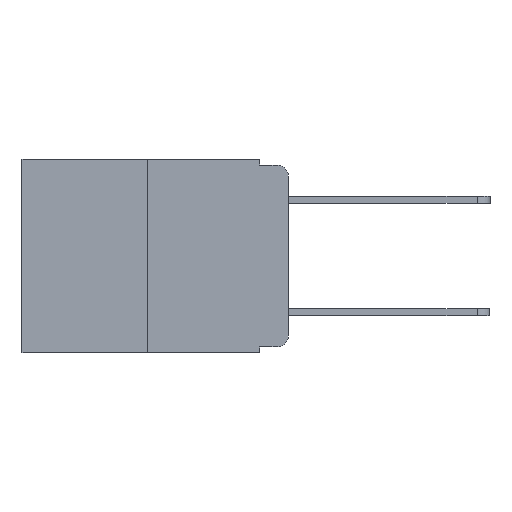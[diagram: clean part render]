
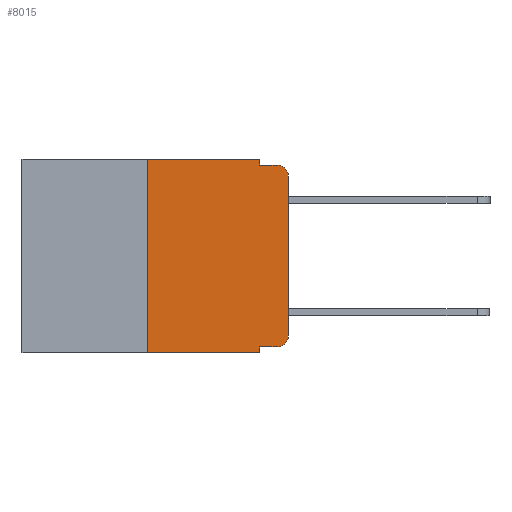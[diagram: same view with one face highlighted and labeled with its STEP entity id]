
A CAD part, left-side view. The second image highlights one B-rep face of the part: STEP entity #8015.
In plain terms, the highlighted planar face has unit normal (-1, 0, 0).
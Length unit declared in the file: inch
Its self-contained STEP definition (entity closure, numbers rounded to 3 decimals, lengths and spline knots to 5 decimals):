
#145 = CARTESIAN_POINT ( 'NONE',  ( 0., 0.02, -0.333 ) ) ;
#206 = DIRECTION ( 'NONE',  ( -1., 0., 0. ) ) ;
#389 = VECTOR ( 'NONE', #14884, 39.37008 ) ;
#493 = EDGE_CURVE ( 'NONE', #17603, #16536, #7752, .T. ) ;
#823 = CARTESIAN_POINT ( 'NONE',  ( 0., 0.051, 0. ) ) ;
#953 = VERTEX_POINT ( 'NONE', #11860 ) ;
#973 = CARTESIAN_POINT ( 'NONE',  ( 0., 0.051, 0. ) ) ;
#1228 = CARTESIAN_POINT ( 'NONE',  ( 0., 0.051, -0.01 ) ) ;
#1438 = LINE ( 'NONE', #3188, #389 ) ;
#1512 = VERTEX_POINT ( 'NONE', #4310 ) ;
#1547 = PLANE ( 'NONE',  #3725 ) ;
#1634 = EDGE_CURVE ( 'NONE', #16536, #2215, #11098, .T. ) ;
#1791 = ORIENTED_EDGE ( 'NONE', *, *, #10806, .T. ) ;
#2012 = VERTEX_POINT ( 'NONE', #9566 ) ;
#2027 = LINE ( 'NONE', #12851, #13285 ) ;
#2215 = VERTEX_POINT ( 'NONE', #7210 ) ;
#2433 = CIRCLE ( 'NONE', #15498, 0.02 ) ;
#2696 = DIRECTION ( 'NONE',  ( 0., 0., -1. ) ) ;
#2817 = LINE ( 'NONE', #3338, #10207 ) ;
#3058 = ORIENTED_EDGE ( 'NONE', *, *, #493, .F. ) ;
#3075 = DIRECTION ( 'NONE',  ( 1., 0., 0. ) ) ;
#3188 = CARTESIAN_POINT ( 'NONE',  ( 0., 0., 0. ) ) ;
#3217 = DIRECTION ( 'NONE',  ( 0., 0., -1. ) ) ;
#3338 = CARTESIAN_POINT ( 'NONE',  ( 0., 0.473, -0.343 ) ) ;
#3560 = EDGE_CURVE ( 'NONE', #15031, #16398, #2027, .T. ) ;
#3725 = AXIS2_PLACEMENT_3D ( 'NONE', #7516, #3075, #13332 ) ;
#3840 = VECTOR ( 'NONE', #14391, 39.37008 ) ;
#4052 = VERTEX_POINT ( 'NONE', #7897 ) ;
#4310 = CARTESIAN_POINT ( 'NONE',  ( 0., 0.02, -0.01 ) ) ;
#4951 = EDGE_CURVE ( 'NONE', #4052, #2012, #2817, .T. ) ;
#5381 = ORIENTED_EDGE ( 'NONE', *, *, #9598, .F. ) ;
#5998 = DIRECTION ( 'NONE',  ( 0., 0., 1. ) ) ;
#7075 = ORIENTED_EDGE ( 'NONE', *, *, #4951, .T. ) ;
#7210 = CARTESIAN_POINT ( 'NONE',  ( 0., 0.051, -0.01 ) ) ;
#7279 = DIRECTION ( 'NONE',  ( -1., 0., 0. ) ) ;
#7516 = CARTESIAN_POINT ( 'NONE',  ( 0., 0.473, 0. ) ) ;
#7700 = VECTOR ( 'NONE', #3217, 39.37008 ) ;
#7752 = LINE ( 'NONE', #12990, #3840 ) ;
#7897 = CARTESIAN_POINT ( 'NONE',  ( 0., 0.25, -0.343 ) ) ;
#8015 = ADVANCED_FACE ( 'NONE', ( #13972 ), #1547, .F. ) ;
#8384 = ORIENTED_EDGE ( 'NONE', *, *, #15509, .T. ) ;
#8617 = ORIENTED_EDGE ( 'NONE', *, *, #1634, .F. ) ;
#8684 = VERTEX_POINT ( 'NONE', #16369 ) ;
#8694 = LINE ( 'NONE', #1228, #12585 ) ;
#8867 = ORIENTED_EDGE ( 'NONE', *, *, #8963, .F. ) ;
#8900 = DIRECTION ( 'NONE',  ( 0., -1., 0. ) ) ;
#8963 = EDGE_CURVE ( 'NONE', #2215, #1512, #8694, .T. ) ;
#9245 = CARTESIAN_POINT ( 'NONE',  ( 0., 0.02, -0.313 ) ) ;
#9375 = LINE ( 'NONE', #10397, #16562 ) ;
#9533 = ORIENTED_EDGE ( 'NONE', *, *, #16787, .T. ) ;
#9566 = CARTESIAN_POINT ( 'NONE',  ( 0., 0.051, -0.343 ) ) ;
#9598 = EDGE_CURVE ( 'NONE', #4052, #17603, #9375, .T. ) ;
#9983 = LINE ( 'NONE', #973, #12927 ) ;
#9994 = DIRECTION ( 'NONE',  ( 0., -1., 0. ) ) ;
#10207 = VECTOR ( 'NONE', #8900, 39.37008 ) ;
#10397 = CARTESIAN_POINT ( 'NONE',  ( 0., 0.25, 0. ) ) ;
#10599 = CARTESIAN_POINT ( 'NONE',  ( 0., 0.051, -0.333 ) ) ;
#10615 = ORIENTED_EDGE ( 'NONE', *, *, #3560, .T. ) ;
#10740 = DIRECTION ( 'NONE',  ( 0., 0., -1. ) ) ;
#10806 = EDGE_CURVE ( 'NONE', #16398, #953, #18041, .T. ) ;
#11098 = LINE ( 'NONE', #823, #7700 ) ;
#11575 = DIRECTION ( 'NONE',  ( 0., -1., 0. ) ) ;
#11860 = CARTESIAN_POINT ( 'NONE',  ( 0., 0., -0.313 ) ) ;
#12585 = VECTOR ( 'NONE', #11575, 39.37008 ) ;
#12851 = CARTESIAN_POINT ( 'NONE',  ( 0., 0.051, -0.333 ) ) ;
#12927 = VECTOR ( 'NONE', #2696, 39.37008 ) ;
#12990 = CARTESIAN_POINT ( 'NONE',  ( 0., 0.473, 0. ) ) ;
#13285 = VECTOR ( 'NONE', #9994, 39.37008 ) ;
#13332 = DIRECTION ( 'NONE',  ( 0., 0., -1. ) ) ;
#13972 = FACE_OUTER_BOUND ( 'NONE', #18704, .T. ) ;
#14391 = DIRECTION ( 'NONE',  ( 0., -1., 0. ) ) ;
#14629 = ORIENTED_EDGE ( 'NONE', *, *, #17834, .F. ) ;
#14884 = DIRECTION ( 'NONE',  ( 0., 0., 1. ) ) ;
#15031 = VERTEX_POINT ( 'NONE', #10599 ) ;
#15498 = AXIS2_PLACEMENT_3D ( 'NONE', #15893, #7279, #17291 ) ;
#15509 = EDGE_CURVE ( 'NONE', #8684, #1512, #2433, .T. ) ;
#15893 = CARTESIAN_POINT ( 'NONE',  ( 0., 0.02, -0.03 ) ) ;
#16369 = CARTESIAN_POINT ( 'NONE',  ( 0., 0., -0.03 ) ) ;
#16398 = VERTEX_POINT ( 'NONE', #145 ) ;
#16536 = VERTEX_POINT ( 'NONE', #17086 ) ;
#16562 = VECTOR ( 'NONE', #5998, 39.37008 ) ;
#16635 = CARTESIAN_POINT ( 'NONE',  ( 0., 0.25, 0. ) ) ;
#16787 = EDGE_CURVE ( 'NONE', #953, #8684, #1438, .T. ) ;
#17086 = CARTESIAN_POINT ( 'NONE',  ( 0., 0.051, 0. ) ) ;
#17291 = DIRECTION ( 'NONE',  ( 0., 0., -1. ) ) ;
#17603 = VERTEX_POINT ( 'NONE', #16635 ) ;
#17834 = EDGE_CURVE ( 'NONE', #15031, #2012, #9983, .T. ) ;
#18041 = CIRCLE ( 'NONE', #18873, 0.02 ) ;
#18704 = EDGE_LOOP ( 'NONE', ( #9533, #8384, #8867, #8617, #3058, #5381, #7075, #14629, #10615, #1791 ) ) ;
#18873 = AXIS2_PLACEMENT_3D ( 'NONE', #9245, #206, #10740 ) ;
